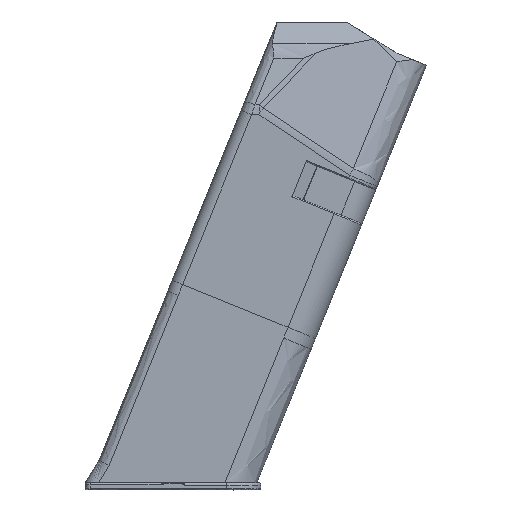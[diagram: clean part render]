
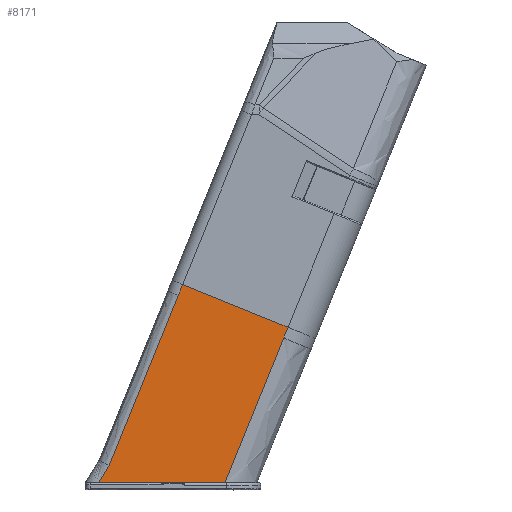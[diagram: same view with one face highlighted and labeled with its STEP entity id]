
A CAD part, top view. The second image highlights one B-rep face of the part: STEP entity #8171.
In plain terms, the highlighted planar face has unit normal (0, 0, 1).
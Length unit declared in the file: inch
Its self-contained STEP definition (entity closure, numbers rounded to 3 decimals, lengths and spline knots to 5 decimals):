
#892=PLANE('',#8748);
#1157=FACE_OUTER_BOUND('',#1601,.T.);
#1601=EDGE_LOOP('',(#5859,#5860,#5861,#5862,#5863,#5864,#5865));
#2025=LINE('',#11392,#2784);
#2026=LINE('',#11403,#2785);
#2035=LINE('',#11439,#2794);
#2093=LINE('',#11634,#2852);
#2094=LINE('',#11638,#2853);
#2095=LINE('',#11640,#2854);
#2096=LINE('',#11641,#2855);
#2784=VECTOR('',#9349,0.3937);
#2785=VECTOR('',#9352,0.3937);
#2794=VECTOR('',#9373,0.3937);
#2852=VECTOR('',#9501,0.3937);
#2853=VECTOR('',#9506,40.55118);
#2854=VECTOR('',#9507,40.48904);
#2855=VECTOR('',#9508,38.6707);
#3795=VERTEX_POINT('',#11386);
#3797=VERTEX_POINT('',#11390);
#3798=VERTEX_POINT('',#11399);
#3800=VERTEX_POINT('',#11402);
#3865=VERTEX_POINT('',#11633);
#3866=VERTEX_POINT('',#11637);
#3867=VERTEX_POINT('',#11639);
#4538=EDGE_CURVE('',#3795,#3797,#2025,.T.);
#4540=EDGE_CURVE('',#3798,#3800,#2026,.T.);
#4554=EDGE_CURVE('',#3800,#3797,#2035,.T.);
#4633=EDGE_CURVE('',#3865,#3795,#2093,.T.);
#4635=EDGE_CURVE('',#3798,#3866,#2094,.T.);
#4636=EDGE_CURVE('',#3866,#3867,#2095,.T.);
#4637=EDGE_CURVE('',#3865,#3867,#2096,.T.);
#5859=ORIENTED_EDGE('',*,*,#4635,.T.);
#5860=ORIENTED_EDGE('',*,*,#4636,.T.);
#5861=ORIENTED_EDGE('',*,*,#4637,.F.);
#5862=ORIENTED_EDGE('',*,*,#4633,.T.);
#5863=ORIENTED_EDGE('',*,*,#4538,.T.);
#5864=ORIENTED_EDGE('',*,*,#4554,.F.);
#5865=ORIENTED_EDGE('',*,*,#4540,.F.);
#8171=ADVANCED_FACE('',(#1157),#892,.T.);
#8748=AXIS2_PLACEMENT_3D('',#11636,#9504,#9505);
#9349=DIRECTION('',(0.376,0.927,0.));
#9352=DIRECTION('',(0.376,0.927,0.));
#9373=DIRECTION('',(0.927,-0.376,0.));
#9501=DIRECTION('',(0.376,0.927,0.));
#9504=DIRECTION('center_axis',(0.,0.,1.));
#9505=DIRECTION('ref_axis',(0.927,-0.376,0.));
#9506=DIRECTION('',(-0.376,-0.927,0.));
#9507=DIRECTION('',(-0.522,-0.853,0.));
#9508=DIRECTION('',(-1.,0.,0.));
#11386=CARTESIAN_POINT('',(2.27768,1.1645,0.45379));
#11390=CARTESIAN_POINT('',(2.31471,1.25569,0.45379));
#11392=CARTESIAN_POINT('',(2.27768,1.1645,0.45379));
#11399=CARTESIAN_POINT('',(1.38854,1.52554,0.45379));
#11402=CARTESIAN_POINT('',(1.42557,1.61673,0.45379));
#11403=CARTESIAN_POINT('',(1.38854,1.52554,0.45379));
#11439=CARTESIAN_POINT('',(1.42557,1.61673,0.45379));
#11633=CARTESIAN_POINT('',(1.78225,-0.0556,0.45379));
#11634=CARTESIAN_POINT('',(2.88671,2.66435,0.45379));
#11636=CARTESIAN_POINT('Origin',(3.00039,2.61272,0.45379));
#11637=CARTESIAN_POINT('',(0.80505,0.08856,0.45379));
#11638=CARTESIAN_POINT('',(0.80834,0.09669,0.45379));
#11639=CARTESIAN_POINT('',(0.71713,-0.0551,0.45379));
#11640=CARTESIAN_POINT('',(0.79286,0.06864,0.45379));
#11641=CARTESIAN_POINT('',(0.70528,-0.0551,0.45379));
